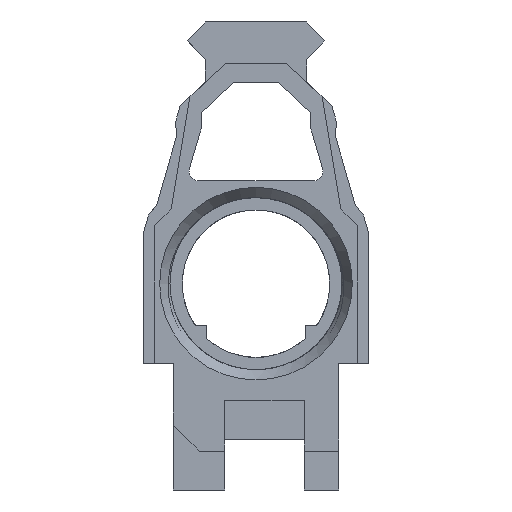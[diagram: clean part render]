
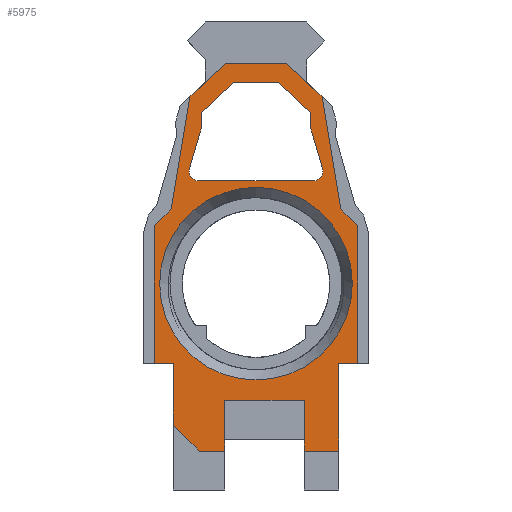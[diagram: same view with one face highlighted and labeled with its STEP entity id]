
A CAD part, front view. The second image highlights one B-rep face of the part: STEP entity #5975.
In plain terms, the highlighted planar face has unit normal (0, -1, 0).
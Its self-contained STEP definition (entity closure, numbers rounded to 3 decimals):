
#85=FACE_BOUND('',#823,.T.);
#86=FACE_BOUND('',#824,.T.);
#170=CIRCLE('',#6282,1.5);
#171=CIRCLE('',#6285,1.5);
#194=CIRCLE('',#6359,14.85);
#507=FACE_OUTER_BOUND('',#822,.T.);
#822=EDGE_LOOP('',(#5284,#5285,#5286,#5287,#5288,#5289,#5290,#5291,#5292,
#5293,#5294,#5295,#5296,#5297,#5298,#5299,#5300,#5301,#5302));
#823=EDGE_LOOP('',(#5303,#5304,#5305,#5306,#5307,#5308,#5309,#5310,#5311,
#5312));
#824=EDGE_LOOP('',(#5313));
#1407=LINE('',#9826,#2136);
#1415=LINE('',#9851,#2144);
#1423=LINE('',#9872,#2152);
#1446=LINE('',#9929,#2175);
#1475=LINE('',#10004,#2204);
#1477=LINE('',#10007,#2206);
#1485=LINE('',#10023,#2214);
#1488=LINE('',#10031,#2217);
#1490=LINE('',#10036,#2219);
#1492=LINE('',#10040,#2221);
#1494=LINE('',#10043,#2223);
#1496=LINE('',#10047,#2225);
#1498=LINE('',#10051,#2227);
#1499=LINE('',#10053,#2228);
#1521=LINE('',#10204,#2250);
#1524=LINE('',#10209,#2253);
#1542=LINE('',#10394,#2271);
#1549=LINE('',#10407,#2278);
#1551=LINE('',#10411,#2280);
#1553=LINE('',#10415,#2282);
#1554=LINE('',#10418,#2283);
#1557=LINE('',#10423,#2286);
#1558=LINE('',#10424,#2287);
#1559=LINE('',#10425,#2288);
#1560=LINE('',#10426,#2289);
#1561=LINE('',#10428,#2290);
#1562=LINE('',#10429,#2291);
#2136=VECTOR('',#7424,10.);
#2144=VECTOR('',#7446,10.);
#2152=VECTOR('',#7462,10.);
#2175=VECTOR('',#7513,10.);
#2204=VECTOR('',#7572,10.);
#2206=VECTOR('',#7574,10.);
#2214=VECTOR('',#7588,10.);
#2217=VECTOR('',#7597,10.);
#2219=VECTOR('',#7601,10.);
#2221=VECTOR('',#7605,10.);
#2223=VECTOR('',#7609,10.);
#2225=VECTOR('',#7613,10.);
#2227=VECTOR('',#7617,10.);
#2228=VECTOR('',#7620,10.);
#2250=VECTOR('',#7686,10.);
#2253=VECTOR('',#7691,10.);
#2271=VECTOR('',#7783,10.);
#2278=VECTOR('',#7794,10.);
#2280=VECTOR('',#7798,10.);
#2282=VECTOR('',#7802,10.);
#2283=VECTOR('',#7805,10.);
#2286=VECTOR('',#7810,10.);
#2287=VECTOR('',#7811,10.);
#2288=VECTOR('',#7812,10.);
#2289=VECTOR('',#7813,10.);
#2290=VECTOR('',#7814,10.);
#2291=VECTOR('',#7815,10.);
#2723=VERTEX_POINT('',#9823);
#2724=VERTEX_POINT('',#9825);
#2733=VERTEX_POINT('',#9848);
#2734=VERTEX_POINT('',#9850);
#2742=VERTEX_POINT('',#9869);
#2743=VERTEX_POINT('',#9871);
#2762=VERTEX_POINT('',#9926);
#2763=VERTEX_POINT('',#9928);
#2786=VERTEX_POINT('',#10002);
#2787=VERTEX_POINT('',#10006);
#2790=VERTEX_POINT('',#10015);
#2791=VERTEX_POINT('',#10017);
#2792=VERTEX_POINT('',#10021);
#2793=VERTEX_POINT('',#10025);
#2794=VERTEX_POINT('',#10027);
#2795=VERTEX_POINT('',#10033);
#2796=VERTEX_POINT('',#10035);
#2797=VERTEX_POINT('',#10039);
#2798=VERTEX_POINT('',#10045);
#2799=VERTEX_POINT('',#10049);
#2830=VERTEX_POINT('',#10201);
#2831=VERTEX_POINT('',#10203);
#2832=VERTEX_POINT('',#10207);
#2844=VERTEX_POINT('',#10393);
#2848=VERTEX_POINT('',#10405);
#2849=VERTEX_POINT('',#10409);
#2850=VERTEX_POINT('',#10413);
#2851=VERTEX_POINT('',#10417);
#2853=VERTEX_POINT('',#10427);
#2854=VERTEX_POINT('',#10430);
#3481=EDGE_CURVE('',#2723,#2724,#1407,.T.);
#3493=EDGE_CURVE('',#2734,#2733,#1415,.T.);
#3503=EDGE_CURVE('',#2743,#2742,#1423,.T.);
#3531=EDGE_CURVE('',#2763,#2762,#1446,.T.);
#3568=EDGE_CURVE('',#2733,#2786,#1475,.T.);
#3570=EDGE_CURVE('',#2787,#2763,#1477,.T.);
#3576=EDGE_CURVE('',#2790,#2791,#170,.T.);
#3579=EDGE_CURVE('',#2790,#2792,#1485,.T.);
#3581=EDGE_CURVE('',#2793,#2794,#171,.T.);
#3583=EDGE_CURVE('',#2793,#2791,#1488,.T.);
#3585=EDGE_CURVE('',#2796,#2795,#1490,.T.);
#3587=EDGE_CURVE('',#2797,#2796,#1492,.T.);
#3589=EDGE_CURVE('',#2792,#2797,#1494,.T.);
#3591=EDGE_CURVE('',#2795,#2798,#1496,.T.);
#3593=EDGE_CURVE('',#2798,#2799,#1498,.T.);
#3594=EDGE_CURVE('',#2799,#2794,#1499,.T.);
#3636=EDGE_CURVE('',#2831,#2830,#1521,.T.);
#3639=EDGE_CURVE('',#2830,#2832,#1524,.T.);
#3675=EDGE_CURVE('',#2844,#2831,#1542,.T.);
#3682=EDGE_CURVE('',#2786,#2848,#1549,.T.);
#3684=EDGE_CURVE('',#2849,#2848,#1551,.T.);
#3686=EDGE_CURVE('',#2832,#2850,#1553,.T.);
#3687=EDGE_CURVE('',#2851,#2762,#1554,.T.);
#3690=EDGE_CURVE('',#2851,#2724,#1557,.T.);
#3691=EDGE_CURVE('',#2723,#2743,#1558,.T.);
#3692=EDGE_CURVE('',#2742,#2734,#1559,.T.);
#3693=EDGE_CURVE('',#2849,#2844,#1560,.T.);
#3694=EDGE_CURVE('',#2853,#2850,#1561,.T.);
#3695=EDGE_CURVE('',#2853,#2787,#1562,.T.);
#3696=EDGE_CURVE('',#2854,#2854,#194,.T.);
#5284=ORIENTED_EDGE('',*,*,#3687,.F.);
#5285=ORIENTED_EDGE('',*,*,#3690,.T.);
#5286=ORIENTED_EDGE('',*,*,#3481,.F.);
#5287=ORIENTED_EDGE('',*,*,#3691,.T.);
#5288=ORIENTED_EDGE('',*,*,#3503,.T.);
#5289=ORIENTED_EDGE('',*,*,#3692,.T.);
#5290=ORIENTED_EDGE('',*,*,#3493,.T.);
#5291=ORIENTED_EDGE('',*,*,#3568,.T.);
#5292=ORIENTED_EDGE('',*,*,#3682,.T.);
#5293=ORIENTED_EDGE('',*,*,#3684,.F.);
#5294=ORIENTED_EDGE('',*,*,#3693,.T.);
#5295=ORIENTED_EDGE('',*,*,#3675,.T.);
#5296=ORIENTED_EDGE('',*,*,#3636,.T.);
#5297=ORIENTED_EDGE('',*,*,#3639,.T.);
#5298=ORIENTED_EDGE('',*,*,#3686,.T.);
#5299=ORIENTED_EDGE('',*,*,#3694,.F.);
#5300=ORIENTED_EDGE('',*,*,#3695,.T.);
#5301=ORIENTED_EDGE('',*,*,#3570,.T.);
#5302=ORIENTED_EDGE('',*,*,#3531,.T.);
#5303=ORIENTED_EDGE('',*,*,#3583,.T.);
#5304=ORIENTED_EDGE('',*,*,#3576,.F.);
#5305=ORIENTED_EDGE('',*,*,#3579,.T.);
#5306=ORIENTED_EDGE('',*,*,#3589,.T.);
#5307=ORIENTED_EDGE('',*,*,#3587,.T.);
#5308=ORIENTED_EDGE('',*,*,#3585,.T.);
#5309=ORIENTED_EDGE('',*,*,#3591,.T.);
#5310=ORIENTED_EDGE('',*,*,#3593,.T.);
#5311=ORIENTED_EDGE('',*,*,#3594,.T.);
#5312=ORIENTED_EDGE('',*,*,#3581,.F.);
#5313=ORIENTED_EDGE('',*,*,#3696,.F.);
#5674=PLANE('',#6358);
#5975=ADVANCED_FACE('',(#507,#85,#86),#5674,.T.);
#6282=AXIS2_PLACEMENT_3D('',#10018,#7582,#7583);
#6285=AXIS2_PLACEMENT_3D('',#10028,#7592,#7593);
#6358=AXIS2_PLACEMENT_3D('',#10422,#7808,#7809);
#6359=AXIS2_PLACEMENT_3D('',#10431,#7816,#7817);
#7424=DIRECTION('',(0.,0.,-1.));
#7446=DIRECTION('',(0.,0.,1.));
#7462=DIRECTION('',(0.,0.,-1.));
#7513=DIRECTION('',(0.,0.,-1.));
#7572=DIRECTION('',(1.,0.,0.));
#7574=DIRECTION('',(1.,0.,0.));
#7582=DIRECTION('center_axis',(0.,-1.,0.));
#7583=DIRECTION('ref_axis',(-0.801,0.,-0.599));
#7588=DIRECTION('',(0.283,0.,0.959));
#7592=DIRECTION('center_axis',(0.,-1.,0.));
#7593=DIRECTION('ref_axis',(0.801,0.,-0.599));
#7597=DIRECTION('',(-1.,0.,0.));
#7601=DIRECTION('',(1.,0.,0.));
#7605=DIRECTION('',(0.729,0.,0.684));
#7609=DIRECTION('',(0.,0.,1.));
#7613=DIRECTION('',(0.729,0.,-0.684));
#7617=DIRECTION('',(0.,0.,-1.));
#7620=DIRECTION('',(0.283,0.,-0.959));
#7686=DIRECTION('',(-1.,0.,0.));
#7691=DIRECTION('',(-0.729,0.,-0.684));
#7783=DIRECTION('',(-0.729,0.,0.684));
#7794=DIRECTION('',(0.,0.,1.));
#7798=DIRECTION('',(0.707,0.,-0.707));
#7802=DIRECTION('',(-0.165,0.,-0.986));
#7805=DIRECTION('',(-0.707,0.,0.707));
#7808=DIRECTION('center_axis',(0.,-1.,0.));
#7809=DIRECTION('ref_axis',(0.,0.,-1.));
#7810=DIRECTION('',(1.,0.,0.));
#7811=DIRECTION('',(1.,0.,0.));
#7812=DIRECTION('',(1.,0.,0.));
#7813=DIRECTION('',(-0.165,0.,0.986));
#7814=DIRECTION('',(0.707,0.,0.707));
#7815=DIRECTION('',(0.,0.,-1.));
#7816=DIRECTION('center_axis',(0.,-1.,0.));
#7817=DIRECTION('ref_axis',(1.,0.,0.));
#9823=CARTESIAN_POINT('',(-4.85,-212.,-14.3));
#9825=CARTESIAN_POINT('',(-4.85,-212.,-22.1));
#9826=CARTESIAN_POINT('',(-4.85,-212.,-6.788));
#9848=CARTESIAN_POINT('',(12.75,-212.,-8.6));
#9850=CARTESIAN_POINT('',(12.75,-212.,-22.1));
#9851=CARTESIAN_POINT('',(12.75,-212.,-6.788));
#9869=CARTESIAN_POINT('',(7.45,-212.,-22.1));
#9871=CARTESIAN_POINT('',(7.45,-212.,-14.3));
#9872=CARTESIAN_POINT('',(7.45,-212.,0.112));
#9926=CARTESIAN_POINT('',(-12.75,-212.,-18.1));
#9928=CARTESIAN_POINT('',(-12.75,-212.,-8.6));
#9929=CARTESIAN_POINT('',(-12.75,-212.,2.963));
#10002=CARTESIAN_POINT('',(15.65,-212.,-8.6));
#10004=CARTESIAN_POINT('',(6.375,-212.,-8.6));
#10006=CARTESIAN_POINT('',(-15.65,-212.,-8.6));
#10007=CARTESIAN_POINT('',(-8.65,-212.,-8.6));
#10015=CARTESIAN_POINT('',(-10.265,-212.,21.481));
#10017=CARTESIAN_POINT('',(-8.826,-212.,19.556));
#10018=CARTESIAN_POINT('Origin',(-8.826,-212.,21.056));
#10021=CARTESIAN_POINT('',(-8.475,-212.,27.55));
#10023=CARTESIAN_POINT('',(-9.903,-212.,22.708));
#10025=CARTESIAN_POINT('',(8.826,-212.,19.556));
#10027=CARTESIAN_POINT('',(10.265,-212.,21.481));
#10028=CARTESIAN_POINT('Origin',(8.826,-212.,21.056));
#10031=CARTESIAN_POINT('',(-5.416,-212.,19.556));
#10033=CARTESIAN_POINT('',(3.5,-212.,34.72));
#10035=CARTESIAN_POINT('',(-3.5,-212.,34.72));
#10036=CARTESIAN_POINT('',(1.75,-212.,34.72));
#10039=CARTESIAN_POINT('',(-8.475,-212.,30.05));
#10040=CARTESIAN_POINT('',(-7.608,-212.,30.863));
#10043=CARTESIAN_POINT('',(-8.475,-212.,22.288));
#10045=CARTESIAN_POINT('',(8.475,-212.,30.05));
#10047=CARTESIAN_POINT('',(10.096,-212.,28.528));
#10049=CARTESIAN_POINT('',(8.475,-212.,27.55));
#10051=CARTESIAN_POINT('',(8.475,-212.,21.038));
#10053=CARTESIAN_POINT('',(11.081,-212.,18.711));
#10201=CARTESIAN_POINT('',(-4.75,-212.,37.65));
#10203=CARTESIAN_POINT('',(4.75,-212.,37.65));
#10204=CARTESIAN_POINT('',(4.75,-212.,37.65));
#10207=CARTESIAN_POINT('',(-10.175,-212.,32.558));
#10209=CARTESIAN_POINT('',(-4.75,-212.,37.65));
#10393=CARTESIAN_POINT('',(10.175,-212.,32.558));
#10394=CARTESIAN_POINT('',(11.676,-212.,31.148));
#10405=CARTESIAN_POINT('',(15.65,-212.,12.648));
#10407=CARTESIAN_POINT('',(15.65,-212.,2.963));
#10409=CARTESIAN_POINT('',(13.065,-212.,15.234));
#10411=CARTESIAN_POINT('',(10.768,-212.,17.53));
#10413=CARTESIAN_POINT('',(-13.065,-212.,15.234));
#10415=CARTESIAN_POINT('',(-11.501,-212.,24.611));
#10417=CARTESIAN_POINT('',(-8.75,-212.,-22.1));
#10418=CARTESIAN_POINT('',(-16.719,-212.,-14.131));
#10422=CARTESIAN_POINT('Origin',(0.,-212.,14.525));
#10423=CARTESIAN_POINT('',(-6.375,-212.,-22.1));
#10424=CARTESIAN_POINT('',(3.075,-212.,-14.3));
#10425=CARTESIAN_POINT('',(3.725,-212.,-22.1));
#10426=CARTESIAN_POINT('',(12.994,-212.,15.657));
#10427=CARTESIAN_POINT('',(-15.65,-212.,12.648));
#10428=CARTESIAN_POINT('',(-10.768,-212.,17.53));
#10429=CARTESIAN_POINT('',(-15.65,-212.,14.587));
#10430=CARTESIAN_POINT('',(-14.85,-212.,3.706));
#10431=CARTESIAN_POINT('Origin',(0.,-212.,3.706));
